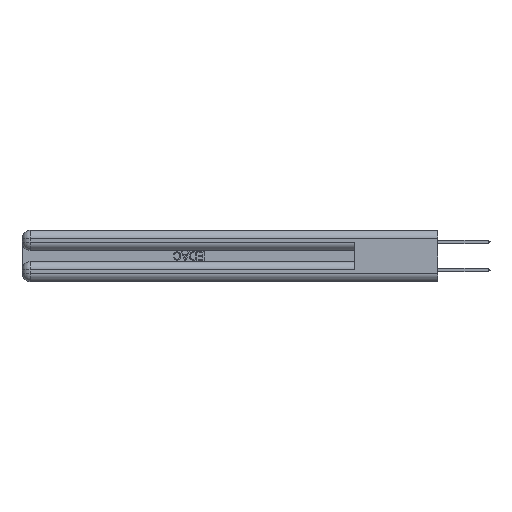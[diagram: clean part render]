
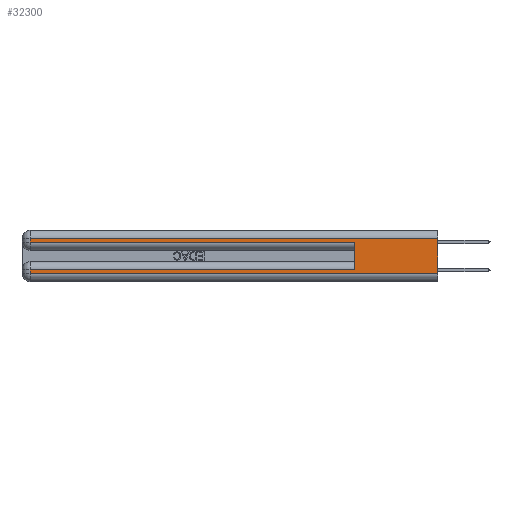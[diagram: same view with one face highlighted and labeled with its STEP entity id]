
A CAD part, left-side view. The second image highlights one B-rep face of the part: STEP entity #32300.
In plain terms, the highlighted planar face has unit normal (-1, 0, 0).
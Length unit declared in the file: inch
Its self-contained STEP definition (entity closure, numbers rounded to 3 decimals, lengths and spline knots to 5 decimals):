
#132 = DIRECTION ( 'NONE',  ( 0., 0., 1. ) ) ;
#389 = DIRECTION ( 'NONE',  ( 1., 0., 0. ) ) ;
#835 = EDGE_CURVE ( 'NONE', #27185, #37802, #5909, .T. ) ;
#1181 = VERTEX_POINT ( 'NONE', #3141 ) ;
#1320 = VECTOR ( 'NONE', #2599, 39.37008 ) ;
#2599 = DIRECTION ( 'NONE',  ( 0., 0., -1. ) ) ;
#2617 = ORIENTED_EDGE ( 'NONE', *, *, #11646, .T. ) ;
#3141 = CARTESIAN_POINT ( 'NONE',  ( 0., 2.94, 0.285 ) ) ;
#4041 = LINE ( 'NONE', #29948, #31409 ) ;
#4155 = CARTESIAN_POINT ( 'NONE',  ( 0., 0., 0.06 ) ) ;
#5909 = LINE ( 'NONE', #34706, #44128 ) ;
#6206 = VECTOR ( 'NONE', #19907, 39.37008 ) ;
#8277 = CARTESIAN_POINT ( 'NONE',  ( 0., 0., 0.285 ) ) ;
#10093 = LINE ( 'NONE', #24929, #1320 ) ;
#10436 = EDGE_CURVE ( 'NONE', #17917, #24970, #4041, .T. ) ;
#11646 = EDGE_CURVE ( 'NONE', #20471, #37682, #22019, .T. ) ;
#12047 = DIRECTION ( 'NONE',  ( 0., -1., 0. ) ) ;
#12354 = CARTESIAN_POINT ( 'NONE',  ( 0., 2.94, 0.37 ) ) ;
#12875 = VECTOR ( 'NONE', #12047, 39.37008 ) ;
#13804 = VECTOR ( 'NONE', #32314, 39.37008 ) ;
#17917 = VERTEX_POINT ( 'NONE', #28415 ) ;
#19111 = CARTESIAN_POINT ( 'NONE',  ( 0., 0., 0.31 ) ) ;
#19852 = CARTESIAN_POINT ( 'NONE',  ( 0., 2.94, 0.31 ) ) ;
#19907 = DIRECTION ( 'NONE',  ( 0., 0., -1. ) ) ;
#20016 = DIRECTION ( 'NONE',  ( 0., 1., 0. ) ) ;
#20471 = VERTEX_POINT ( 'NONE', #20580 ) ;
#20580 = CARTESIAN_POINT ( 'NONE',  ( 0., 2.94, 0.06 ) ) ;
#21187 = EDGE_CURVE ( 'NONE', #17917, #46514, #23709, .T. ) ;
#21324 = ORIENTED_EDGE ( 'NONE', *, *, #36719, .T. ) ;
#21872 = ORIENTED_EDGE ( 'NONE', *, *, #835, .T. ) ;
#22019 = LINE ( 'NONE', #38506, #40479 ) ;
#22738 = PLANE ( 'NONE',  #39842 ) ;
#23709 = LINE ( 'NONE', #46845, #13804 ) ;
#24039 = EDGE_CURVE ( 'NONE', #37802, #1181, #37006, .T. ) ;
#24173 = ORIENTED_EDGE ( 'NONE', *, *, #24039, .T. ) ;
#24929 = CARTESIAN_POINT ( 'NONE',  ( 0., 2.94, 0.37 ) ) ;
#24970 = VERTEX_POINT ( 'NONE', #42372 ) ;
#25969 = LINE ( 'NONE', #47604, #43231 ) ;
#26452 = DIRECTION ( 'NONE',  ( 0., 0., -1. ) ) ;
#27185 = VERTEX_POINT ( 'NONE', #19111 ) ;
#27667 = ORIENTED_EDGE ( 'NONE', *, *, #10436, .F. ) ;
#28415 = CARTESIAN_POINT ( 'NONE',  ( 0., 0.6, 0.085 ) ) ;
#29388 = ORIENTED_EDGE ( 'NONE', *, *, #43291, .F. ) ;
#29948 = CARTESIAN_POINT ( 'NONE',  ( 0., 0.6, 0.145 ) ) ;
#30011 = DIRECTION ( 'NONE',  ( 0., 0., -1. ) ) ;
#31409 = VECTOR ( 'NONE', #132, 39.37008 ) ;
#32058 = CARTESIAN_POINT ( 'NONE',  ( 0., 2.94, 0.085 ) ) ;
#32300 = ADVANCED_FACE ( 'NONE', ( #47735 ), #22738, .F. ) ;
#32314 = DIRECTION ( 'NONE',  ( 0., 1., 0. ) ) ;
#34706 = CARTESIAN_POINT ( 'NONE',  ( 0., 0., 0.31 ) ) ;
#36719 = EDGE_CURVE ( 'NONE', #46514, #20471, #10093, .T. ) ;
#37006 = LINE ( 'NONE', #12354, #6206 ) ;
#37433 = CARTESIAN_POINT ( 'NONE',  ( 0., 0., 0.37 ) ) ;
#37682 = VERTEX_POINT ( 'NONE', #4155 ) ;
#37802 = VERTEX_POINT ( 'NONE', #19852 ) ;
#38506 = CARTESIAN_POINT ( 'NONE',  ( 0., 0., 0.06 ) ) ;
#39842 = AXIS2_PLACEMENT_3D ( 'NONE', #37433, #389, #26452 ) ;
#40479 = VECTOR ( 'NONE', #45825, 39.37008 ) ;
#42372 = CARTESIAN_POINT ( 'NONE',  ( 0., 0.6, 0.285 ) ) ;
#42376 = LINE ( 'NONE', #8277, #12875 ) ;
#42907 = EDGE_LOOP ( 'NONE', ( #29388, #21872, #24173, #43752, #27667, #47187, #21324, #2617 ) ) ;
#43231 = VECTOR ( 'NONE', #30011, 39.37008 ) ;
#43291 = EDGE_CURVE ( 'NONE', #27185, #37682, #25969, .T. ) ;
#43752 = ORIENTED_EDGE ( 'NONE', *, *, #46910, .T. ) ;
#44128 = VECTOR ( 'NONE', #20016, 39.37008 ) ;
#45825 = DIRECTION ( 'NONE',  ( 0., -1., 0. ) ) ;
#46514 = VERTEX_POINT ( 'NONE', #32058 ) ;
#46845 = CARTESIAN_POINT ( 'NONE',  ( 0., 0., 0.085 ) ) ;
#46910 = EDGE_CURVE ( 'NONE', #1181, #24970, #42376, .T. ) ;
#47187 = ORIENTED_EDGE ( 'NONE', *, *, #21187, .T. ) ;
#47604 = CARTESIAN_POINT ( 'NONE',  ( 0., 0., 0.37 ) ) ;
#47735 = FACE_OUTER_BOUND ( 'NONE', #42907, .T. ) ;
